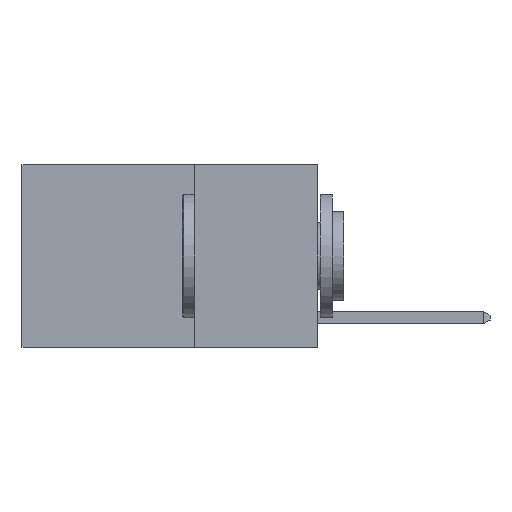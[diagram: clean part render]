
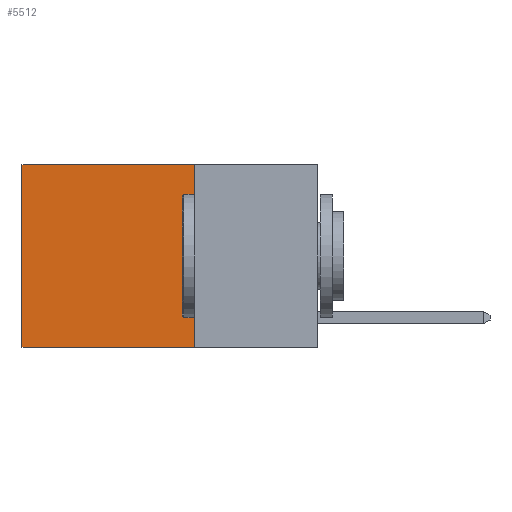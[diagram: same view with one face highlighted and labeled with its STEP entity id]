
A CAD part, left-side view. The second image highlights one B-rep face of the part: STEP entity #5512.
In plain terms, the highlighted planar face has unit normal (-1, 0, 0).
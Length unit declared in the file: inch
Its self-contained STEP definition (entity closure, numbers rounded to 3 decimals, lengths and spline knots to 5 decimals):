
#178 = VERTEX_POINT ( 'NONE', #3150 ) ;
#360 = LINE ( 'NONE', #1778, #2499 ) ;
#470 = DIRECTION ( 'NONE',  ( 0., 0., -1. ) ) ;
#544 = DIRECTION ( 'NONE',  ( 1., 0., 0. ) ) ;
#559 = AXIS2_PLACEMENT_3D ( 'NONE', #6313, #544, #5605 ) ;
#1006 = FACE_OUTER_BOUND ( 'NONE', #1653, .T. ) ;
#1170 = VERTEX_POINT ( 'NONE', #8511 ) ;
#1456 = EDGE_CURVE ( 'NONE', #178, #5179, #2096, .T. ) ;
#1633 = VECTOR ( 'NONE', #6315, 39.37008 ) ;
#1653 = EDGE_LOOP ( 'NONE', ( #4466, #4617, #4997, #5710 ) ) ;
#1778 = CARTESIAN_POINT ( 'NONE',  ( 0.2625, 0.25, -0.37 ) ) ;
#1782 = VECTOR ( 'NONE', #470, 39.37008 ) ;
#1884 = CARTESIAN_POINT ( 'NONE',  ( 0.2625, 0.25, 0. ) ) ;
#2096 = LINE ( 'NONE', #5919, #1633 ) ;
#2494 = CARTESIAN_POINT ( 'NONE',  ( 0.2625, 0.6, 0. ) ) ;
#2499 = VECTOR ( 'NONE', #6163, 39.37008 ) ;
#3150 = CARTESIAN_POINT ( 'NONE',  ( 0.2625, 0.25, 0. ) ) ;
#3318 = LINE ( 'NONE', #1884, #1782 ) ;
#3777 = LINE ( 'NONE', #2494, #7185 ) ;
#3824 = CARTESIAN_POINT ( 'NONE',  ( 0.2625, 0.6, 0. ) ) ;
#4466 = ORIENTED_EDGE ( 'NONE', *, *, #7491, .T. ) ;
#4617 = ORIENTED_EDGE ( 'NONE', *, *, #4709, .F. ) ;
#4709 = EDGE_CURVE ( 'NONE', #1170, #7468, #360, .T. ) ;
#4816 = EDGE_CURVE ( 'NONE', #178, #1170, #3318, .T. ) ;
#4896 = PLANE ( 'NONE',  #559 ) ;
#4997 = ORIENTED_EDGE ( 'NONE', *, *, #4816, .F. ) ;
#5179 = VERTEX_POINT ( 'NONE', #3824 ) ;
#5381 = CARTESIAN_POINT ( 'NONE',  ( 0.2625, 0.6, -0.37 ) ) ;
#5512 = ADVANCED_FACE ( 'NONE', ( #1006 ), #4896, .F. ) ;
#5605 = DIRECTION ( 'NONE',  ( 0., 0., -1. ) ) ;
#5710 = ORIENTED_EDGE ( 'NONE', *, *, #1456, .T. ) ;
#5919 = CARTESIAN_POINT ( 'NONE',  ( 0.2625, 0.25, 0. ) ) ;
#6163 = DIRECTION ( 'NONE',  ( 0., 1., 0. ) ) ;
#6313 = CARTESIAN_POINT ( 'NONE',  ( 0.2625, 0.25, 0. ) ) ;
#6315 = DIRECTION ( 'NONE',  ( 0., 1., 0. ) ) ;
#7185 = VECTOR ( 'NONE', #8214, 39.37008 ) ;
#7468 = VERTEX_POINT ( 'NONE', #5381 ) ;
#7491 = EDGE_CURVE ( 'NONE', #5179, #7468, #3777, .T. ) ;
#8214 = DIRECTION ( 'NONE',  ( 0., 0., -1. ) ) ;
#8511 = CARTESIAN_POINT ( 'NONE',  ( 0.2625, 0.25, -0.37 ) ) ;
